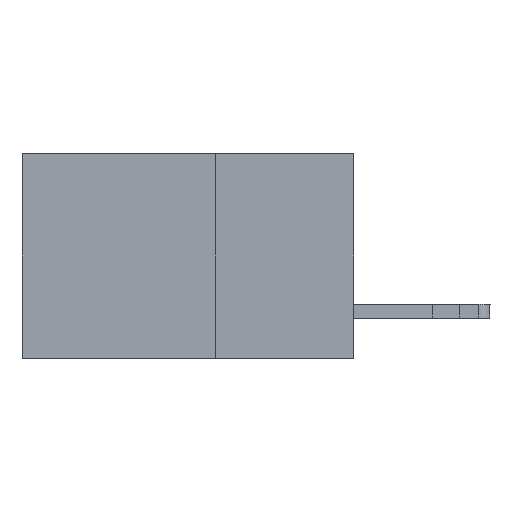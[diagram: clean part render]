
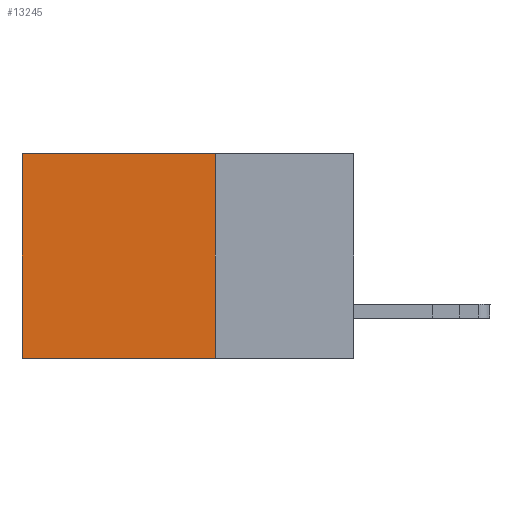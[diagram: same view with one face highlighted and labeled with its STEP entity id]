
A CAD part, left-side view. The second image highlights one B-rep face of the part: STEP entity #13245.
In plain terms, the highlighted planar face has unit normal (-1, 0, 0).
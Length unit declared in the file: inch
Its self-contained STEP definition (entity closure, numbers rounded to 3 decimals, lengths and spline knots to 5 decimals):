
#1171 = VERTEX_POINT ( 'NONE', #16182 ) ;
#1575 = ORIENTED_EDGE ( 'NONE', *, *, #26901, .T. ) ;
#1879 = DIRECTION ( 'NONE',  ( 0., 0., -1. ) ) ;
#2443 = FACE_OUTER_BOUND ( 'NONE', #26169, .T. ) ;
#2568 = DIRECTION ( 'NONE',  ( 0., 0., -1. ) ) ;
#3590 = ORIENTED_EDGE ( 'NONE', *, *, #13035, .T. ) ;
#3708 = LINE ( 'NONE', #25543, #30153 ) ;
#3884 = ORIENTED_EDGE ( 'NONE', *, *, #5361, .F. ) ;
#4677 = DIRECTION ( 'NONE',  ( 0., 0., -1. ) ) ;
#5361 = EDGE_CURVE ( 'NONE', #7197, #1171, #14797, .T. ) ;
#5884 = CARTESIAN_POINT ( 'NONE',  ( 0.2875, 0.6, 0. ) ) ;
#7197 = VERTEX_POINT ( 'NONE', #7380 ) ;
#7369 = CARTESIAN_POINT ( 'NONE',  ( 0.2875, 0.25, 0. ) ) ;
#7380 = CARTESIAN_POINT ( 'NONE',  ( 0.2875, 0.25, 0. ) ) ;
#7798 = CARTESIAN_POINT ( 'NONE',  ( 0.2875, 0.6, -0.37 ) ) ;
#8643 = EDGE_CURVE ( 'NONE', #1171, #16622, #12796, .T. ) ;
#8974 = VECTOR ( 'NONE', #9821, 39.37008 ) ;
#9821 = DIRECTION ( 'NONE',  ( 0., 1., 0. ) ) ;
#10295 = ORIENTED_EDGE ( 'NONE', *, *, #8643, .F. ) ;
#12165 = CARTESIAN_POINT ( 'NONE',  ( 0.2875, 0.25, 0. ) ) ;
#12796 = LINE ( 'NONE', #21907, #8974 ) ;
#13035 = EDGE_CURVE ( 'NONE', #7197, #24444, #3708, .T. ) ;
#13245 = ADVANCED_FACE ( 'NONE', ( #2443 ), #26807, .F. ) ;
#14353 = AXIS2_PLACEMENT_3D ( 'NONE', #12165, #26483, #4677 ) ;
#14797 = LINE ( 'NONE', #7369, #18063 ) ;
#15954 = DIRECTION ( 'NONE',  ( 0., 1., 0. ) ) ;
#16182 = CARTESIAN_POINT ( 'NONE',  ( 0.2875, 0.25, -0.37 ) ) ;
#16622 = VERTEX_POINT ( 'NONE', #7798 ) ;
#18063 = VECTOR ( 'NONE', #2568, 39.37008 ) ;
#20663 = VECTOR ( 'NONE', #1879, 39.37008 ) ;
#21907 = CARTESIAN_POINT ( 'NONE',  ( 0.2875, 0.25, -0.37 ) ) ;
#23880 = LINE ( 'NONE', #26240, #20663 ) ;
#24444 = VERTEX_POINT ( 'NONE', #5884 ) ;
#25543 = CARTESIAN_POINT ( 'NONE',  ( 0.2875, 0.25, 0. ) ) ;
#26169 = EDGE_LOOP ( 'NONE', ( #1575, #10295, #3884, #3590 ) ) ;
#26240 = CARTESIAN_POINT ( 'NONE',  ( 0.2875, 0.6, 0. ) ) ;
#26483 = DIRECTION ( 'NONE',  ( 1., 0., 0. ) ) ;
#26807 = PLANE ( 'NONE',  #14353 ) ;
#26901 = EDGE_CURVE ( 'NONE', #24444, #16622, #23880, .T. ) ;
#30153 = VECTOR ( 'NONE', #15954, 39.37008 ) ;
